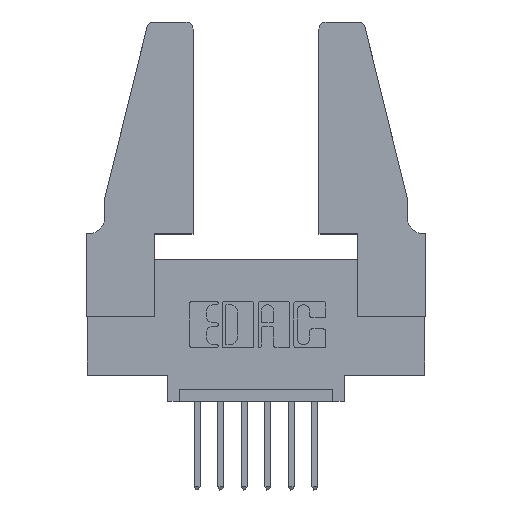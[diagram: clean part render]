
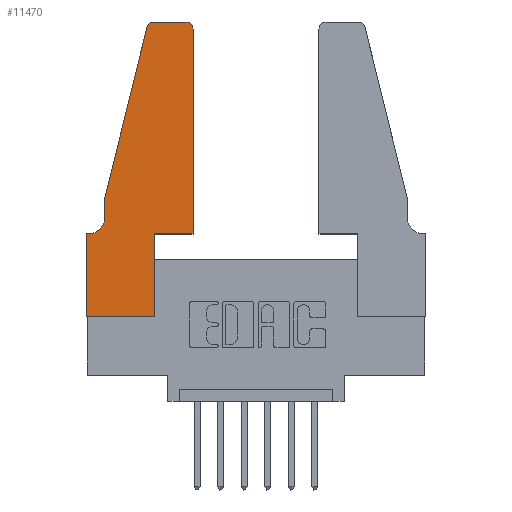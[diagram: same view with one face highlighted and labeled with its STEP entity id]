
A CAD part, top view. The second image highlights one B-rep face of the part: STEP entity #11470.
In plain terms, the highlighted planar face has unit normal (0, 0, 1).
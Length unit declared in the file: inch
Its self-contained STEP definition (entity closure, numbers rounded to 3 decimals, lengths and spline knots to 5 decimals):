
#50 = CARTESIAN_POINT ( 'NONE',  ( 0., 0., 0.37 ) ) ;
#71 = ORIENTED_EDGE ( 'NONE', *, *, #5155, .T. ) ;
#434 = DIRECTION ( 'NONE',  ( 1., 0., 0. ) ) ;
#442 = CARTESIAN_POINT ( 'NONE',  ( 0.4505, 0.35, 0.37 ) ) ;
#566 = DIRECTION ( 'NONE',  ( 0., 0., 1. ) ) ;
#608 = VERTEX_POINT ( 'NONE', #5373 ) ;
#807 = EDGE_CURVE ( 'NONE', #10212, #8572, #6603, .T. ) ;
#1009 = AXIS2_PLACEMENT_3D ( 'NONE', #3267, #566, #7640 ) ;
#1051 = VERTEX_POINT ( 'NONE', #11447 ) ;
#1146 = EDGE_CURVE ( 'NONE', #1539, #5275, #10289, .T. ) ;
#1270 = EDGE_CURVE ( 'NONE', #5365, #3905, #4107, .T. ) ;
#1275 = LINE ( 'NONE', #5882, #5504 ) ;
#1276 = AXIS2_PLACEMENT_3D ( 'NONE', #8810, #3408, #10703 ) ;
#1294 = ORIENTED_EDGE ( 'NONE', *, *, #8316, .T. ) ;
#1351 = ORIENTED_EDGE ( 'NONE', *, *, #2829, .T. ) ;
#1354 = ORIENTED_EDGE ( 'NONE', *, *, #7747, .T. ) ;
#1502 = CARTESIAN_POINT ( 'NONE',  ( 0.0755, 0.42, 0.37 ) ) ;
#1516 = CARTESIAN_POINT ( 'NONE',  ( 0.0755, 0.5, 0.37 ) ) ;
#1539 = VERTEX_POINT ( 'NONE', #1502 ) ;
#1578 = EDGE_CURVE ( 'NONE', #608, #10212, #9850, .T. ) ;
#1656 = ORIENTED_EDGE ( 'NONE', *, *, #807, .T. ) ;
#2228 = VECTOR ( 'NONE', #6843, 39.37008 ) ;
#2314 = DIRECTION ( 'NONE',  ( 1., 0., 0. ) ) ;
#2469 = CARTESIAN_POINT ( 'NONE',  ( 0.0055, 0.35, 0.37 ) ) ;
#2609 = CARTESIAN_POINT ( 'NONE',  ( 0., 0.35, 0.37 ) ) ;
#2829 = EDGE_CURVE ( 'NONE', #1051, #608, #3791, .T. ) ;
#2845 = CARTESIAN_POINT ( 'NONE',  ( 0.4505, 1.22, 0.37 ) ) ;
#2960 = DIRECTION ( 'NONE',  ( 0., -1., 0. ) ) ;
#3153 = VECTOR ( 'NONE', #2960, 39.37008 ) ;
#3256 = ORIENTED_EDGE ( 'NONE', *, *, #4468, .T. ) ;
#3267 = CARTESIAN_POINT ( 'NONE',  ( 0.4205, 1.22, 0.37 ) ) ;
#3408 = DIRECTION ( 'NONE',  ( 0., 0., 1. ) ) ;
#3517 = DIRECTION ( 'NONE',  ( 0., 0., -1. ) ) ;
#3521 = VECTOR ( 'NONE', #434, 39.37008 ) ;
#3770 = CARTESIAN_POINT ( 'NONE',  ( 0., 0., 0.37 ) ) ;
#3791 = LINE ( 'NONE', #11451, #2228 ) ;
#3822 = VECTOR ( 'NONE', #9105, 39.37008 ) ;
#3859 = CIRCLE ( 'NONE', #1276, 0.03 ) ;
#3905 = VERTEX_POINT ( 'NONE', #3770 ) ;
#4107 = LINE ( 'NONE', #50, #3822 ) ;
#4447 = DIRECTION ( 'NONE',  ( -1., 0., 0. ) ) ;
#4468 = EDGE_CURVE ( 'NONE', #8572, #9511, #8099, .T. ) ;
#4867 = AXIS2_PLACEMENT_3D ( 'NONE', #11560, #3517, #4447 ) ;
#5070 = EDGE_CURVE ( 'NONE', #9511, #6997, #11333, .T. ) ;
#5155 = EDGE_CURVE ( 'NONE', #8498, #11307, #6380, .T. ) ;
#5275 = VERTEX_POINT ( 'NONE', #2469 ) ;
#5365 = VERTEX_POINT ( 'NONE', #2609 ) ;
#5373 = CARTESIAN_POINT ( 'NONE',  ( 0.2865, 0.35, 0.37 ) ) ;
#5405 = CARTESIAN_POINT ( 'NONE',  ( 0.284, 1.25, 0.37 ) ) ;
#5504 = VECTOR ( 'NONE', #11316, 39.37008 ) ;
#5582 = CARTESIAN_POINT ( 'NONE',  ( 0.4205, 1.25, 0.37 ) ) ;
#5882 = CARTESIAN_POINT ( 'NONE',  ( 0.0755, 0.35, 0.37 ) ) ;
#6232 = VECTOR ( 'NONE', #11023, 39.37008 ) ;
#6380 = LINE ( 'NONE', #8582, #11476 ) ;
#6603 = LINE ( 'NONE', #8411, #9159 ) ;
#6843 = DIRECTION ( 'NONE',  ( 0., 1., 0. ) ) ;
#6851 = FACE_OUTER_BOUND ( 'NONE', #7693, .T. ) ;
#6863 = AXIS2_PLACEMENT_3D ( 'NONE', #9584, #11343, #2314 ) ;
#6997 = VERTEX_POINT ( 'NONE', #5405 ) ;
#7640 = DIRECTION ( 'NONE',  ( 1., 0., 0. ) ) ;
#7693 = EDGE_LOOP ( 'NONE', ( #8103, #1294, #71, #1354, #9219, #11628, #9229, #11366, #1351, #8457, #1656, #3256 ) ) ;
#7747 = EDGE_CURVE ( 'NONE', #11307, #1539, #8085, .T. ) ;
#7922 = LINE ( 'NONE', #8513, #10737 ) ;
#8085 = LINE ( 'NONE', #8351, #3153 ) ;
#8099 = CIRCLE ( 'NONE', #1009, 0.03 ) ;
#8103 = ORIENTED_EDGE ( 'NONE', *, *, #5070, .T. ) ;
#8316 = EDGE_CURVE ( 'NONE', #6997, #8498, #3859, .T. ) ;
#8351 = CARTESIAN_POINT ( 'NONE',  ( 0.0755, 0.5, 0.37 ) ) ;
#8411 = CARTESIAN_POINT ( 'NONE',  ( 0.4505, 0.35, 0.37 ) ) ;
#8457 = ORIENTED_EDGE ( 'NONE', *, *, #1578, .T. ) ;
#8498 = VERTEX_POINT ( 'NONE', #8621 ) ;
#8513 = CARTESIAN_POINT ( 'NONE',  ( 0., 0., 0.37 ) ) ;
#8572 = VERTEX_POINT ( 'NONE', #2845 ) ;
#8582 = CARTESIAN_POINT ( 'NONE',  ( 0.0755, 0.5, 0.37 ) ) ;
#8596 = DIRECTION ( 'NONE',  ( 1., 0., 0. ) ) ;
#8621 = CARTESIAN_POINT ( 'NONE',  ( 0.25487, 1.22718, 0.37 ) ) ;
#8630 = EDGE_CURVE ( 'NONE', #3905, #1051, #7922, .T. ) ;
#8810 = CARTESIAN_POINT ( 'NONE',  ( 0.284, 1.22, 0.37 ) ) ;
#9105 = DIRECTION ( 'NONE',  ( 0., -1., 0. ) ) ;
#9159 = VECTOR ( 'NONE', #9309, 39.37008 ) ;
#9219 = ORIENTED_EDGE ( 'NONE', *, *, #1146, .T. ) ;
#9229 = ORIENTED_EDGE ( 'NONE', *, *, #1270, .T. ) ;
#9309 = DIRECTION ( 'NONE',  ( 0., 1., 0. ) ) ;
#9470 = DIRECTION ( 'NONE',  ( -0.239, -0.971, 0. ) ) ;
#9511 = VERTEX_POINT ( 'NONE', #5582 ) ;
#9584 = CARTESIAN_POINT ( 'NONE',  ( 0., 0.35, 0.37 ) ) ;
#9774 = EDGE_CURVE ( 'NONE', #5275, #5365, #1275, .T. ) ;
#9850 = LINE ( 'NONE', #10395, #3521 ) ;
#10095 = CARTESIAN_POINT ( 'NONE',  ( 0.2605, 1.25, 0.37 ) ) ;
#10212 = VERTEX_POINT ( 'NONE', #442 ) ;
#10289 = CIRCLE ( 'NONE', #4867, 0.07 ) ;
#10395 = CARTESIAN_POINT ( 'NONE',  ( 0.4505, 0.35, 0.37 ) ) ;
#10703 = DIRECTION ( 'NONE',  ( 1., 0., 0. ) ) ;
#10737 = VECTOR ( 'NONE', #8596, 39.37008 ) ;
#11023 = DIRECTION ( 'NONE',  ( -1., 0., 0. ) ) ;
#11307 = VERTEX_POINT ( 'NONE', #1516 ) ;
#11316 = DIRECTION ( 'NONE',  ( -1., 0., 0. ) ) ;
#11333 = LINE ( 'NONE', #10095, #6232 ) ;
#11343 = DIRECTION ( 'NONE',  ( 0., 0., 1. ) ) ;
#11366 = ORIENTED_EDGE ( 'NONE', *, *, #8630, .T. ) ;
#11447 = CARTESIAN_POINT ( 'NONE',  ( 0.2865, 0., 0.37 ) ) ;
#11451 = CARTESIAN_POINT ( 'NONE',  ( 0.2865, 0.35, 0.37 ) ) ;
#11457 = PLANE ( 'NONE',  #6863 ) ;
#11470 = ADVANCED_FACE ( 'NONE', ( #6851 ), #11457, .T. ) ;
#11476 = VECTOR ( 'NONE', #9470, 39.37008 ) ;
#11560 = CARTESIAN_POINT ( 'NONE',  ( 0.0055, 0.42, 0.37 ) ) ;
#11628 = ORIENTED_EDGE ( 'NONE', *, *, #9774, .T. ) ;
